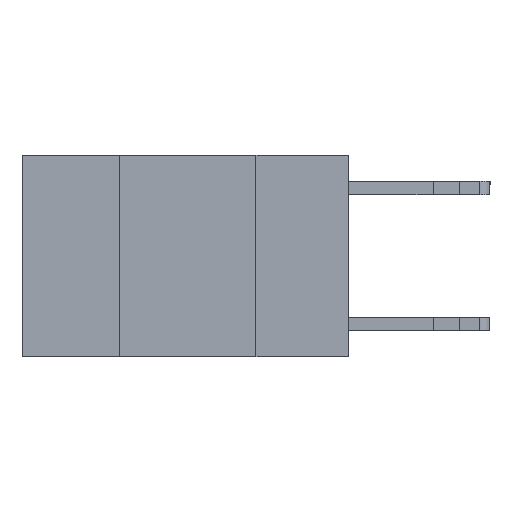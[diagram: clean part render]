
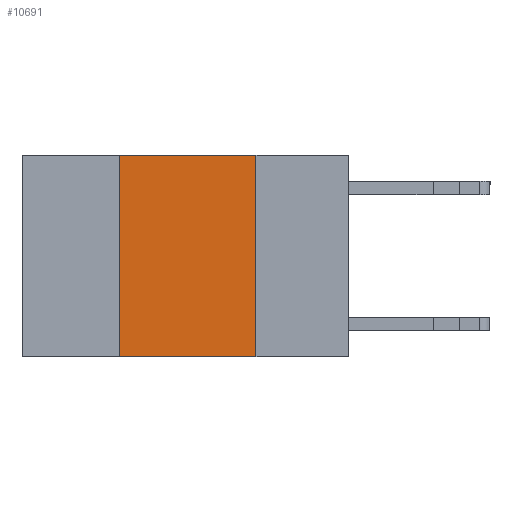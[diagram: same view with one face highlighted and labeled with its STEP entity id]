
A CAD part, left-side view. The second image highlights one B-rep face of the part: STEP entity #10691.
In plain terms, the highlighted planar face has unit normal (-1, 0, 0).
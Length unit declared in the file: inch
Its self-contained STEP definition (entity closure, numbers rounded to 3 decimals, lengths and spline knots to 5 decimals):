
#336 = DIRECTION ( 'NONE',  ( 1., 0., 0. ) ) ;
#937 = VERTEX_POINT ( 'NONE', #7546 ) ;
#1553 = CARTESIAN_POINT ( 'NONE',  ( 0., 0.17, 0. ) ) ;
#2208 = VERTEX_POINT ( 'NONE', #10537 ) ;
#2620 = CARTESIAN_POINT ( 'NONE',  ( 0., 0.42, 0. ) ) ;
#2856 = CARTESIAN_POINT ( 'NONE',  ( 0., 0.6, 0. ) ) ;
#2884 = EDGE_CURVE ( 'NONE', #9358, #11450, #4462, .T. ) ;
#3174 = DIRECTION ( 'NONE',  ( 0., 0., -1. ) ) ;
#3716 = EDGE_CURVE ( 'NONE', #11450, #2208, #11939, .T. ) ;
#3888 = CARTESIAN_POINT ( 'NONE',  ( 0., 0.42, -0.37 ) ) ;
#4132 = CARTESIAN_POINT ( 'NONE',  ( 0., 0.6, 0. ) ) ;
#4462 = LINE ( 'NONE', #2620, #8674 ) ;
#5165 = FACE_OUTER_BOUND ( 'NONE', #9787, .T. ) ;
#5241 = EDGE_CURVE ( 'NONE', #9358, #937, #9729, .T. ) ;
#6552 = DIRECTION ( 'NONE',  ( 0., -1., 0. ) ) ;
#7172 = EDGE_CURVE ( 'NONE', #2208, #937, #11708, .T. ) ;
#7370 = VECTOR ( 'NONE', #10761, 39.37008 ) ;
#7546 = CARTESIAN_POINT ( 'NONE',  ( 0., 0.17, -0.37 ) ) ;
#8674 = VECTOR ( 'NONE', #8889, 39.37008 ) ;
#8889 = DIRECTION ( 'NONE',  ( 0., 0., 1. ) ) ;
#9358 = VERTEX_POINT ( 'NONE', #3888 ) ;
#9372 = CARTESIAN_POINT ( 'NONE',  ( 0., 0.42, 0. ) ) ;
#9405 = ORIENTED_EDGE ( 'NONE', *, *, #3716, .F. ) ;
#9729 = LINE ( 'NONE', #10824, #7370 ) ;
#9787 = EDGE_LOOP ( 'NONE', ( #11000, #9405, #10619, #11569 ) ) ;
#9877 = DIRECTION ( 'NONE',  ( 0., 0., -1. ) ) ;
#9961 = AXIS2_PLACEMENT_3D ( 'NONE', #4132, #336, #3174 ) ;
#10537 = CARTESIAN_POINT ( 'NONE',  ( 0., 0.17, 0. ) ) ;
#10619 = ORIENTED_EDGE ( 'NONE', *, *, #2884, .F. ) ;
#10691 = ADVANCED_FACE ( 'NONE', ( #5165 ), #11531, .F. ) ;
#10761 = DIRECTION ( 'NONE',  ( 0., -1., 0. ) ) ;
#10824 = CARTESIAN_POINT ( 'NONE',  ( 0., 0.6, -0.37 ) ) ;
#11000 = ORIENTED_EDGE ( 'NONE', *, *, #7172, .F. ) ;
#11024 = VECTOR ( 'NONE', #6552, 39.37008 ) ;
#11450 = VERTEX_POINT ( 'NONE', #9372 ) ;
#11531 = PLANE ( 'NONE',  #9961 ) ;
#11569 = ORIENTED_EDGE ( 'NONE', *, *, #5241, .T. ) ;
#11616 = VECTOR ( 'NONE', #9877, 39.37008 ) ;
#11708 = LINE ( 'NONE', #1553, #11616 ) ;
#11939 = LINE ( 'NONE', #2856, #11024 ) ;
